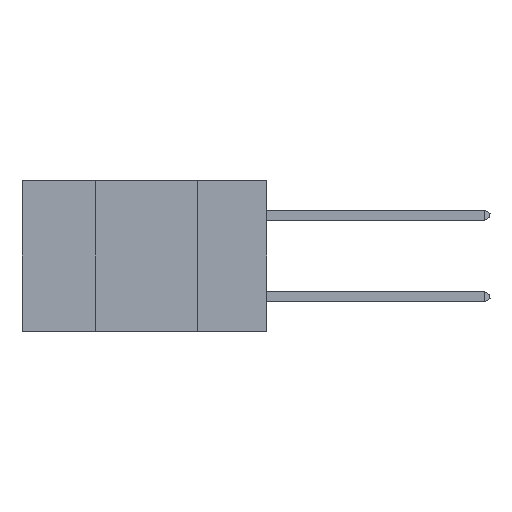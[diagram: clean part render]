
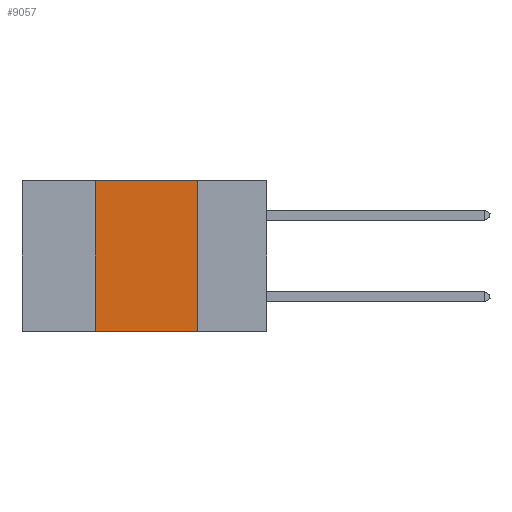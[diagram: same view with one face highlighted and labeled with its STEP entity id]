
A CAD part, left-side view. The second image highlights one B-rep face of the part: STEP entity #9057.
In plain terms, the highlighted planar face has unit normal (-1, 0, 0).
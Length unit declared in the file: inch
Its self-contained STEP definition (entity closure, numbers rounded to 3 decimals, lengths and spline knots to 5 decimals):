
#627 = VECTOR ( 'NONE', #1023, 39.37008 ) ;
#732 = VERTEX_POINT ( 'NONE', #6906 ) ;
#979 = LINE ( 'NONE', #1138, #2669 ) ;
#1023 = DIRECTION ( 'NONE',  ( 0., 0., -1. ) ) ;
#1138 = CARTESIAN_POINT ( 'NONE',  ( 0., 0.42, 0. ) ) ;
#1620 = EDGE_CURVE ( 'NONE', #3843, #3390, #8141, .T. ) ;
#2027 = DIRECTION ( 'NONE',  ( 0., -1., 0. ) ) ;
#2669 = VECTOR ( 'NONE', #6947, 39.37008 ) ;
#2925 = CARTESIAN_POINT ( 'NONE',  ( 0., 0.6, -0.37 ) ) ;
#3385 = FACE_OUTER_BOUND ( 'NONE', #5459, .T. ) ;
#3390 = VERTEX_POINT ( 'NONE', #6262 ) ;
#3718 = DIRECTION ( 'NONE',  ( 1., 0., 0. ) ) ;
#3843 = VERTEX_POINT ( 'NONE', #6012 ) ;
#4419 = PLANE ( 'NONE',  #10308 ) ;
#5125 = ORIENTED_EDGE ( 'NONE', *, *, #5622, .F. ) ;
#5459 = EDGE_LOOP ( 'NONE', ( #9054, #9200, #5125, #6107 ) ) ;
#5563 = LINE ( 'NONE', #2925, #5915 ) ;
#5622 = EDGE_CURVE ( 'NONE', #7116, #3843, #979, .T. ) ;
#5915 = VECTOR ( 'NONE', #2027, 39.37008 ) ;
#5950 = CARTESIAN_POINT ( 'NONE',  ( 0., 0.17, 0. ) ) ;
#6012 = CARTESIAN_POINT ( 'NONE',  ( 0., 0.42, 0. ) ) ;
#6099 = DIRECTION ( 'NONE',  ( 0., -1., 0. ) ) ;
#6107 = ORIENTED_EDGE ( 'NONE', *, *, #10236, .T. ) ;
#6262 = CARTESIAN_POINT ( 'NONE',  ( 0., 0.17, 0. ) ) ;
#6906 = CARTESIAN_POINT ( 'NONE',  ( 0., 0.17, -0.37 ) ) ;
#6947 = DIRECTION ( 'NONE',  ( 0., 0., 1. ) ) ;
#7116 = VERTEX_POINT ( 'NONE', #9776 ) ;
#7802 = LINE ( 'NONE', #5950, #627 ) ;
#8141 = LINE ( 'NONE', #8627, #8272 ) ;
#8272 = VECTOR ( 'NONE', #6099, 39.37008 ) ;
#8627 = CARTESIAN_POINT ( 'NONE',  ( 0., 0.6, 0. ) ) ;
#8732 = CARTESIAN_POINT ( 'NONE',  ( 0., 0.6, 0. ) ) ;
#9054 = ORIENTED_EDGE ( 'NONE', *, *, #10078, .F. ) ;
#9057 = ADVANCED_FACE ( 'NONE', ( #3385 ), #4419, .F. ) ;
#9200 = ORIENTED_EDGE ( 'NONE', *, *, #1620, .F. ) ;
#9617 = DIRECTION ( 'NONE',  ( 0., 0., -1. ) ) ;
#9776 = CARTESIAN_POINT ( 'NONE',  ( 0., 0.42, -0.37 ) ) ;
#10078 = EDGE_CURVE ( 'NONE', #3390, #732, #7802, .T. ) ;
#10236 = EDGE_CURVE ( 'NONE', #7116, #732, #5563, .T. ) ;
#10308 = AXIS2_PLACEMENT_3D ( 'NONE', #8732, #3718, #9617 ) ;
